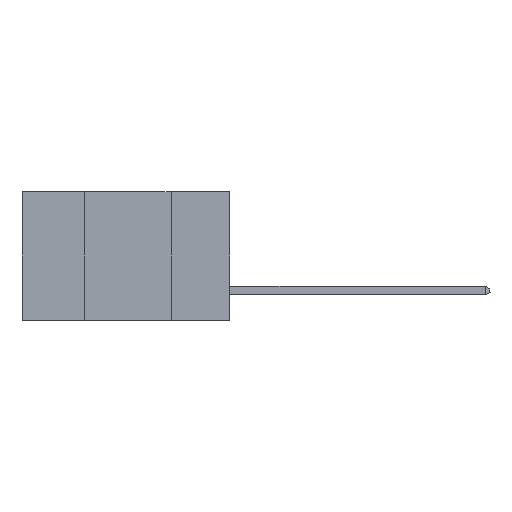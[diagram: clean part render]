
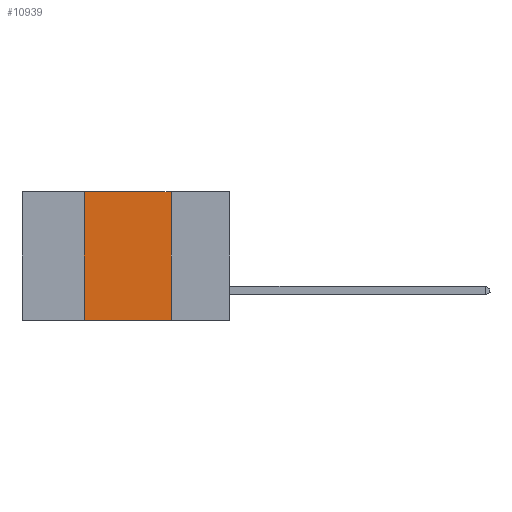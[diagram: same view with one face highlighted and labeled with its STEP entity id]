
A CAD part, left-side view. The second image highlights one B-rep face of the part: STEP entity #10939.
In plain terms, the highlighted planar face has unit normal (-1, 0, 0).
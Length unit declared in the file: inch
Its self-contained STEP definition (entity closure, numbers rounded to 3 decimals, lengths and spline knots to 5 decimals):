
#475 = VECTOR ( 'NONE', #12063, 39.37008 ) ;
#625 = LINE ( 'NONE', #19736, #4825 ) ;
#1135 = VECTOR ( 'NONE', #1932, 39.37008 ) ;
#1932 = DIRECTION ( 'NONE',  ( 0., -1., 0. ) ) ;
#3011 = VERTEX_POINT ( 'NONE', #13056 ) ;
#3080 = VECTOR ( 'NONE', #16704, 39.37008 ) ;
#3449 = AXIS2_PLACEMENT_3D ( 'NONE', #21574, #7196, #9084 ) ;
#4825 = VECTOR ( 'NONE', #21364, 39.37008 ) ;
#6758 = LINE ( 'NONE', #16629, #3080 ) ;
#6825 = CARTESIAN_POINT ( 'NONE',  ( 0., 0.6, -0.37 ) ) ;
#7196 = DIRECTION ( 'NONE',  ( 1., 0., 0. ) ) ;
#8552 = ORIENTED_EDGE ( 'NONE', *, *, #18022, .F. ) ;
#9084 = DIRECTION ( 'NONE',  ( 0., 0., -1. ) ) ;
#9727 = VERTEX_POINT ( 'NONE', #11195 ) ;
#10939 = ADVANCED_FACE ( 'NONE', ( #22479 ), #19789, .F. ) ;
#11195 = CARTESIAN_POINT ( 'NONE',  ( 0., 0.17, -0.37 ) ) ;
#11338 = EDGE_CURVE ( 'NONE', #3011, #9727, #625, .T. ) ;
#11371 = CARTESIAN_POINT ( 'NONE',  ( 0., 0.42, 0. ) ) ;
#12063 = DIRECTION ( 'NONE',  ( 0., -1., 0. ) ) ;
#12073 = EDGE_CURVE ( 'NONE', #16644, #3011, #14057, .T. ) ;
#13056 = CARTESIAN_POINT ( 'NONE',  ( 0., 0.17, 0. ) ) ;
#13730 = ORIENTED_EDGE ( 'NONE', *, *, #11338, .F. ) ;
#14057 = LINE ( 'NONE', #17915, #1135 ) ;
#14695 = EDGE_CURVE ( 'NONE', #19016, #9727, #21483, .T. ) ;
#15938 = ORIENTED_EDGE ( 'NONE', *, *, #12073, .F. ) ;
#16629 = CARTESIAN_POINT ( 'NONE',  ( 0., 0.42, 0. ) ) ;
#16644 = VERTEX_POINT ( 'NONE', #11371 ) ;
#16704 = DIRECTION ( 'NONE',  ( 0., 0., 1. ) ) ;
#17915 = CARTESIAN_POINT ( 'NONE',  ( 0., 0.6, 0. ) ) ;
#18022 = EDGE_CURVE ( 'NONE', #19016, #16644, #6758, .T. ) ;
#19016 = VERTEX_POINT ( 'NONE', #20986 ) ;
#19736 = CARTESIAN_POINT ( 'NONE',  ( 0., 0.17, 0. ) ) ;
#19740 = EDGE_LOOP ( 'NONE', ( #13730, #15938, #8552, #22525 ) ) ;
#19789 = PLANE ( 'NONE',  #3449 ) ;
#20986 = CARTESIAN_POINT ( 'NONE',  ( 0., 0.42, -0.37 ) ) ;
#21364 = DIRECTION ( 'NONE',  ( 0., 0., -1. ) ) ;
#21483 = LINE ( 'NONE', #6825, #475 ) ;
#21574 = CARTESIAN_POINT ( 'NONE',  ( 0., 0.6, 0. ) ) ;
#22479 = FACE_OUTER_BOUND ( 'NONE', #19740, .T. ) ;
#22525 = ORIENTED_EDGE ( 'NONE', *, *, #14695, .T. ) ;
